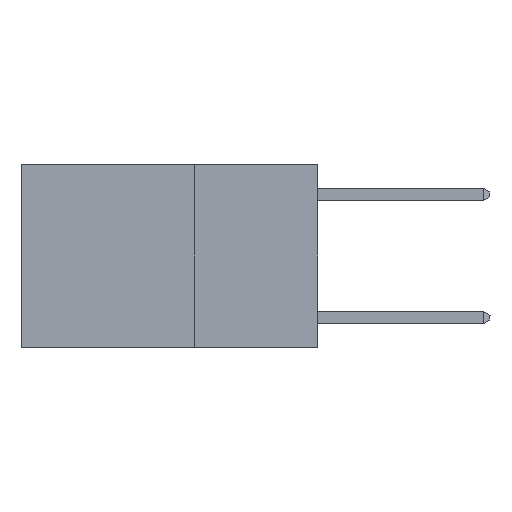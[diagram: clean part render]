
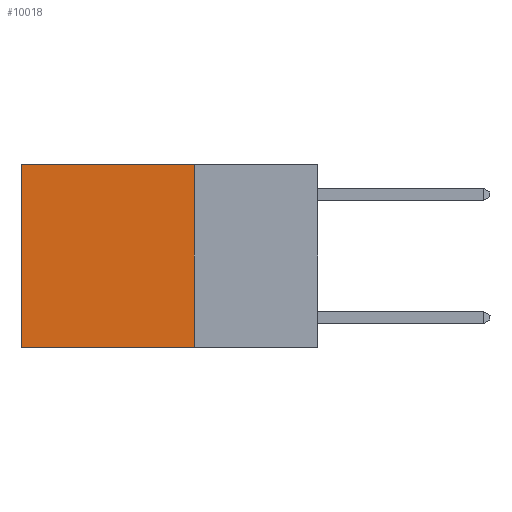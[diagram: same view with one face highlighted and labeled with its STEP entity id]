
A CAD part, left-side view. The second image highlights one B-rep face of the part: STEP entity #10018.
In plain terms, the highlighted planar face has unit normal (-1, 0, 0).
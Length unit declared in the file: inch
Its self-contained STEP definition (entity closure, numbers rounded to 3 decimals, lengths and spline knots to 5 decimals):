
#12 = CARTESIAN_POINT ( 'NONE',  ( 0.2625, 0.25, -0.37 ) ) ;
#261 = LINE ( 'NONE', #9761, #14238 ) ;
#739 = ORIENTED_EDGE ( 'NONE', *, *, #6200, .F. ) ;
#870 = DIRECTION ( 'NONE',  ( 0., 0., -1. ) ) ;
#1277 = CARTESIAN_POINT ( 'NONE',  ( 0.2625, 0.6, 0. ) ) ;
#1356 = VECTOR ( 'NONE', #3233, 39.37008 ) ;
#2948 = LINE ( 'NONE', #14568, #10969 ) ;
#3233 = DIRECTION ( 'NONE',  ( 0., 1., 0. ) ) ;
#4672 = LINE ( 'NONE', #7888, #1356 ) ;
#5398 = CARTESIAN_POINT ( 'NONE',  ( 0.2625, 0.25, 0. ) ) ;
#5424 = CARTESIAN_POINT ( 'NONE',  ( 0.2625, 0.25, 0. ) ) ;
#5774 = ORIENTED_EDGE ( 'NONE', *, *, #6671, .T. ) ;
#6200 = EDGE_CURVE ( 'NONE', #9797, #9795, #2948, .T. ) ;
#6562 = DIRECTION ( 'NONE',  ( 1., 0., 0. ) ) ;
#6671 = EDGE_CURVE ( 'NONE', #9797, #10548, #4672, .T. ) ;
#6784 = EDGE_CURVE ( 'NONE', #10548, #13689, #261, .T. ) ;
#6919 = CARTESIAN_POINT ( 'NONE',  ( 0.2625, 0.6, -0.37 ) ) ;
#6953 = DIRECTION ( 'NONE',  ( 0., 1., 0. ) ) ;
#7417 = DIRECTION ( 'NONE',  ( 0., 0., -1. ) ) ;
#7864 = FACE_OUTER_BOUND ( 'NONE', #9642, .T. ) ;
#7888 = CARTESIAN_POINT ( 'NONE',  ( 0.2625, 0.25, 0. ) ) ;
#7985 = ORIENTED_EDGE ( 'NONE', *, *, #11123, .F. ) ;
#8773 = ORIENTED_EDGE ( 'NONE', *, *, #6784, .T. ) ;
#9642 = EDGE_LOOP ( 'NONE', ( #8773, #7985, #739, #5774 ) ) ;
#9761 = CARTESIAN_POINT ( 'NONE',  ( 0.2625, 0.6, 0. ) ) ;
#9795 = VERTEX_POINT ( 'NONE', #14390 ) ;
#9797 = VERTEX_POINT ( 'NONE', #5424 ) ;
#9951 = LINE ( 'NONE', #12, #10666 ) ;
#10018 = ADVANCED_FACE ( 'NONE', ( #7864 ), #10961, .F. ) ;
#10548 = VERTEX_POINT ( 'NONE', #1277 ) ;
#10666 = VECTOR ( 'NONE', #6953, 39.37008 ) ;
#10960 = AXIS2_PLACEMENT_3D ( 'NONE', #5398, #6562, #870 ) ;
#10961 = PLANE ( 'NONE',  #10960 ) ;
#10969 = VECTOR ( 'NONE', #14516, 39.37008 ) ;
#11123 = EDGE_CURVE ( 'NONE', #9795, #13689, #9951, .T. ) ;
#13689 = VERTEX_POINT ( 'NONE', #6919 ) ;
#14238 = VECTOR ( 'NONE', #7417, 39.37008 ) ;
#14390 = CARTESIAN_POINT ( 'NONE',  ( 0.2625, 0.25, -0.37 ) ) ;
#14516 = DIRECTION ( 'NONE',  ( 0., 0., -1. ) ) ;
#14568 = CARTESIAN_POINT ( 'NONE',  ( 0.2625, 0.25, 0. ) ) ;
